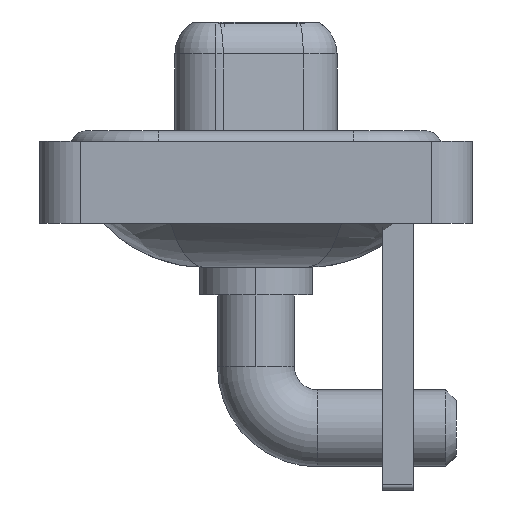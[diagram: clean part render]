
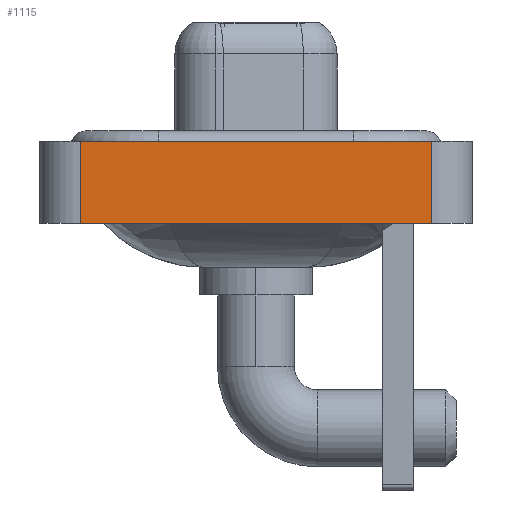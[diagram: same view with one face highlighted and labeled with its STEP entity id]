
A CAD part, left-side view. The second image highlights one B-rep face of the part: STEP entity #1115.
In plain terms, the highlighted planar face has unit normal (-1, 0, 0).
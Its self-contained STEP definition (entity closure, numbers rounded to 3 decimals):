
#87 = CARTESIAN_POINT ( 'NONE',  ( -7.35, 8.55, -3.6 ) ) ;
#247 = DIRECTION ( 'NONE',  ( 0., 0., 1. ) ) ;
#476 = CARTESIAN_POINT ( 'NONE',  ( -7.35, -8.55, -3.6 ) ) ;
#1115 = ADVANCED_FACE ( 'NONE', ( #7787 ), #12229, .T. ) ;
#1118 = EDGE_CURVE ( 'NONE', #2246, #2884, #11737, .T. ) ;
#1463 = EDGE_CURVE ( 'NONE', #15659, #2884, #5197, .T. ) ;
#1831 = CARTESIAN_POINT ( 'NONE',  ( -7.35, 8.55, 0.4 ) ) ;
#2246 = VERTEX_POINT ( 'NONE', #476 ) ;
#2443 = CARTESIAN_POINT ( 'NONE',  ( -7.35, -8.55, -3.6 ) ) ;
#2639 = VECTOR ( 'NONE', #14242, 1000. ) ;
#2765 = CARTESIAN_POINT ( 'NONE',  ( -7.35, 8.55, -3.6 ) ) ;
#2884 = VERTEX_POINT ( 'NONE', #8854 ) ;
#3026 = CARTESIAN_POINT ( 'NONE',  ( -7.35, -8.55, -3.6 ) ) ;
#3078 = EDGE_CURVE ( 'NONE', #6063, #15659, #12068, .T. ) ;
#3511 = EDGE_CURVE ( 'NONE', #6063, #2246, #4868, .T. ) ;
#3627 = ORIENTED_EDGE ( 'NONE', *, *, #3511, .T. ) ;
#4868 = LINE ( 'NONE', #13279, #6803 ) ;
#5197 = LINE ( 'NONE', #7584, #2639 ) ;
#6063 = VERTEX_POINT ( 'NONE', #2765 ) ;
#6803 = VECTOR ( 'NONE', #9160, 1000. ) ;
#7456 = ORIENTED_EDGE ( 'NONE', *, *, #3078, .F. ) ;
#7584 = CARTESIAN_POINT ( 'NONE',  ( -7.35, -8.55, 0.4 ) ) ;
#7787 = FACE_OUTER_BOUND ( 'NONE', #9200, .T. ) ;
#8364 = VECTOR ( 'NONE', #9608, 1000. ) ;
#8854 = CARTESIAN_POINT ( 'NONE',  ( -7.35, -8.55, 0.4 ) ) ;
#9110 = DIRECTION ( 'NONE',  ( -1., 0., 0. ) ) ;
#9160 = DIRECTION ( 'NONE',  ( 0., -1., 0. ) ) ;
#9200 = EDGE_LOOP ( 'NONE', ( #10703, #12451, #7456, #3627 ) ) ;
#9608 = DIRECTION ( 'NONE',  ( 0., 0., 1. ) ) ;
#10703 = ORIENTED_EDGE ( 'NONE', *, *, #1118, .T. ) ;
#11737 = LINE ( 'NONE', #3026, #8364 ) ;
#12068 = LINE ( 'NONE', #87, #14898 ) ;
#12229 = PLANE ( 'NONE',  #13668 ) ;
#12239 = DIRECTION ( 'NONE',  ( 0., 0., 1. ) ) ;
#12451 = ORIENTED_EDGE ( 'NONE', *, *, #1463, .F. ) ;
#13279 = CARTESIAN_POINT ( 'NONE',  ( -7.35, -8.55, -3.6 ) ) ;
#13668 = AXIS2_PLACEMENT_3D ( 'NONE', #2443, #9110, #247 ) ;
#14242 = DIRECTION ( 'NONE',  ( 0., -1., 0. ) ) ;
#14898 = VECTOR ( 'NONE', #12239, 1000. ) ;
#15659 = VERTEX_POINT ( 'NONE', #1831 ) ;
